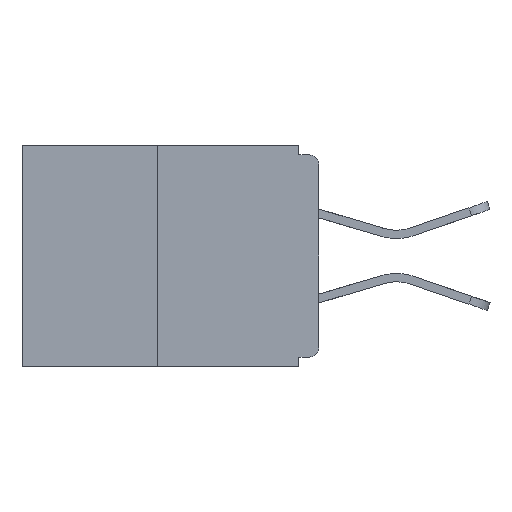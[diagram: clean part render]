
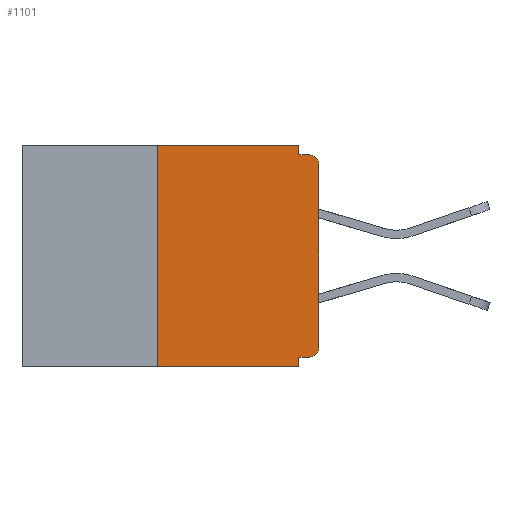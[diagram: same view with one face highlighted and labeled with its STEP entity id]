
A CAD part, left-side view. The second image highlights one B-rep face of the part: STEP entity #1101.
In plain terms, the highlighted planar face has unit normal (-1, 0, 0).
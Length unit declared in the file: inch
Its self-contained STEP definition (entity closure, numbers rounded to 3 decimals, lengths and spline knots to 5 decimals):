
#229 = DIRECTION ( 'NONE',  ( 0., -1., 0. ) ) ;
#390 = VERTEX_POINT ( 'NONE', #6318 ) ;
#526 = DIRECTION ( 'NONE',  ( 0., 0., -1. ) ) ;
#672 = ORIENTED_EDGE ( 'NONE', *, *, #6109, .T. ) ;
#775 = ORIENTED_EDGE ( 'NONE', *, *, #15537, .F. ) ;
#808 = CARTESIAN_POINT ( 'NONE',  ( 0., 0.015, -0.03 ) ) ;
#964 = CARTESIAN_POINT ( 'NONE',  ( 0., 0., -0.015 ) ) ;
#1101 = ADVANCED_FACE ( 'NONE', ( #4792 ), #8001, .F. ) ;
#1537 = CARTESIAN_POINT ( 'NONE',  ( 0., 0.031, -0.328 ) ) ;
#1588 = VECTOR ( 'NONE', #13655, 39.37008 ) ;
#1796 = AXIS2_PLACEMENT_3D ( 'NONE', #3731, #3792, #9859 ) ;
#1824 = CARTESIAN_POINT ( 'NONE',  ( 0., 0.46, -0.343 ) ) ;
#2751 = VERTEX_POINT ( 'NONE', #13097 ) ;
#2825 = DIRECTION ( 'NONE',  ( 0., 1., 0. ) ) ;
#3127 = ORIENTED_EDGE ( 'NONE', *, *, #17266, .F. ) ;
#3731 = CARTESIAN_POINT ( 'NONE',  ( 0., 0.015, -0.313 ) ) ;
#3792 = DIRECTION ( 'NONE',  ( -1., 0., 0. ) ) ;
#3875 = CARTESIAN_POINT ( 'NONE',  ( 0., 0.25, 0. ) ) ;
#3879 = CARTESIAN_POINT ( 'NONE',  ( 0., 0., -0.03 ) ) ;
#4792 = FACE_OUTER_BOUND ( 'NONE', #13504, .T. ) ;
#5000 = EDGE_CURVE ( 'NONE', #6305, #13812, #11726, .T. ) ;
#5344 = DIRECTION ( 'NONE',  ( 0., 0., 1. ) ) ;
#5410 = LINE ( 'NONE', #1824, #6108 ) ;
#6108 = VECTOR ( 'NONE', #229, 39.37008 ) ;
#6109 = EDGE_CURVE ( 'NONE', #8718, #11494, #8840, .T. ) ;
#6305 = VERTEX_POINT ( 'NONE', #1537 ) ;
#6318 = CARTESIAN_POINT ( 'NONE',  ( 0., 0.25, -0.343 ) ) ;
#6991 = CARTESIAN_POINT ( 'NONE',  ( 0., 0.46, 0. ) ) ;
#7013 = VERTEX_POINT ( 'NONE', #18155 ) ;
#7227 = ORIENTED_EDGE ( 'NONE', *, *, #16971, .F. ) ;
#7544 = VERTEX_POINT ( 'NONE', #17927 ) ;
#7629 = CARTESIAN_POINT ( 'NONE',  ( 0., 0., -0.328 ) ) ;
#7901 = VECTOR ( 'NONE', #2825, 39.37008 ) ;
#8001 = PLANE ( 'NONE',  #16305 ) ;
#8286 = DIRECTION ( 'NONE',  ( -1., 0., 0. ) ) ;
#8718 = VERTEX_POINT ( 'NONE', #3879 ) ;
#8767 = LINE ( 'NONE', #6991, #1588 ) ;
#8840 = CIRCLE ( 'NONE', #13991, 0.015 ) ;
#9657 = LINE ( 'NONE', #12313, #12482 ) ;
#9805 = DIRECTION ( 'NONE',  ( 0., 0., -1. ) ) ;
#9859 = DIRECTION ( 'NONE',  ( 0., 0., -1. ) ) ;
#10138 = CARTESIAN_POINT ( 'NONE',  ( 0., 0.015, -0.015 ) ) ;
#10162 = DIRECTION ( 'NONE',  ( 0., -1., 0. ) ) ;
#10571 = LINE ( 'NONE', #16982, #18842 ) ;
#10744 = LINE ( 'NONE', #7629, #7901 ) ;
#11494 = VERTEX_POINT ( 'NONE', #10138 ) ;
#11726 = LINE ( 'NONE', #15261, #12179 ) ;
#12179 = VECTOR ( 'NONE', #526, 39.37008 ) ;
#12313 = CARTESIAN_POINT ( 'NONE',  ( 0., 0.031, 0. ) ) ;
#12432 = ORIENTED_EDGE ( 'NONE', *, *, #17404, .T. ) ;
#12482 = VECTOR ( 'NONE', #12895, 39.37008 ) ;
#12733 = DIRECTION ( 'NONE',  ( 0., 0., 1. ) ) ;
#12895 = DIRECTION ( 'NONE',  ( 0., 0., -1. ) ) ;
#13037 = CARTESIAN_POINT ( 'NONE',  ( 0., 0.015, -0.328 ) ) ;
#13097 = CARTESIAN_POINT ( 'NONE',  ( 0., 0.031, 0. ) ) ;
#13184 = ORIENTED_EDGE ( 'NONE', *, *, #15910, .F. ) ;
#13380 = VECTOR ( 'NONE', #10162, 39.37008 ) ;
#13476 = EDGE_CURVE ( 'NONE', #390, #13812, #5410, .T. ) ;
#13504 = EDGE_LOOP ( 'NONE', ( #13184, #7227, #18823, #17688, #775, #14122, #12432, #672, #13854, #3127 ) ) ;
#13655 = DIRECTION ( 'NONE',  ( 0., -1., 0. ) ) ;
#13812 = VERTEX_POINT ( 'NONE', #18502 ) ;
#13854 = ORIENTED_EDGE ( 'NONE', *, *, #18402, .F. ) ;
#13907 = EDGE_CURVE ( 'NONE', #15105, #15523, #15796, .T. ) ;
#13991 = AXIS2_PLACEMENT_3D ( 'NONE', #808, #8286, #9805 ) ;
#14122 = ORIENTED_EDGE ( 'NONE', *, *, #13907, .T. ) ;
#14630 = LINE ( 'NONE', #3875, #18642 ) ;
#15105 = VERTEX_POINT ( 'NONE', #13037 ) ;
#15261 = CARTESIAN_POINT ( 'NONE',  ( 0., 0.031, -0.343 ) ) ;
#15513 = LINE ( 'NONE', #964, #13380 ) ;
#15523 = VERTEX_POINT ( 'NONE', #19388 ) ;
#15537 = EDGE_CURVE ( 'NONE', #15105, #6305, #10744, .T. ) ;
#15796 = CIRCLE ( 'NONE', #1796, 0.015 ) ;
#15910 = EDGE_CURVE ( 'NONE', #7013, #2751, #8767, .T. ) ;
#16305 = AXIS2_PLACEMENT_3D ( 'NONE', #18555, #17181, #18694 ) ;
#16971 = EDGE_CURVE ( 'NONE', #390, #7013, #14630, .T. ) ;
#16982 = CARTESIAN_POINT ( 'NONE',  ( 0., 0., 0. ) ) ;
#17181 = DIRECTION ( 'NONE',  ( 1., 0., 0. ) ) ;
#17266 = EDGE_CURVE ( 'NONE', #2751, #7544, #9657, .T. ) ;
#17404 = EDGE_CURVE ( 'NONE', #15523, #8718, #10571, .T. ) ;
#17688 = ORIENTED_EDGE ( 'NONE', *, *, #5000, .F. ) ;
#17927 = CARTESIAN_POINT ( 'NONE',  ( 0., 0.031, -0.015 ) ) ;
#18155 = CARTESIAN_POINT ( 'NONE',  ( 0., 0.25, 0. ) ) ;
#18402 = EDGE_CURVE ( 'NONE', #7544, #11494, #15513, .T. ) ;
#18502 = CARTESIAN_POINT ( 'NONE',  ( 0., 0.031, -0.343 ) ) ;
#18555 = CARTESIAN_POINT ( 'NONE',  ( 0., 0.46, 0. ) ) ;
#18642 = VECTOR ( 'NONE', #5344, 39.37008 ) ;
#18694 = DIRECTION ( 'NONE',  ( 0., 0., -1. ) ) ;
#18823 = ORIENTED_EDGE ( 'NONE', *, *, #13476, .T. ) ;
#18842 = VECTOR ( 'NONE', #12733, 39.37008 ) ;
#19388 = CARTESIAN_POINT ( 'NONE',  ( 0., 0., -0.313 ) ) ;
